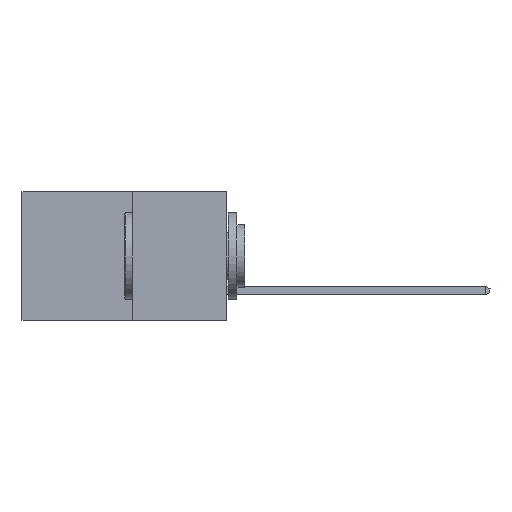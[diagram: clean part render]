
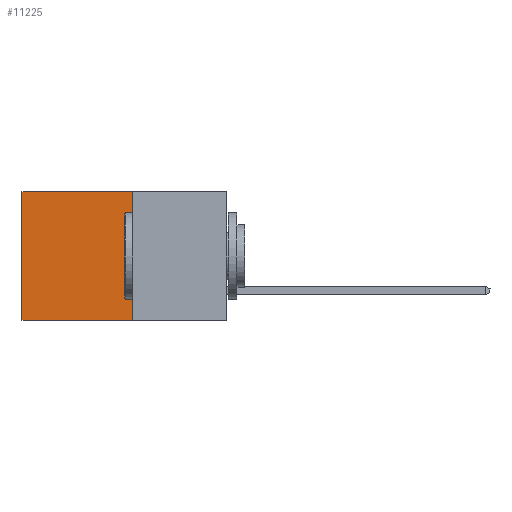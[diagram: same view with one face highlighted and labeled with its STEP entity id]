
A CAD part, left-side view. The second image highlights one B-rep face of the part: STEP entity #11225.
In plain terms, the highlighted planar face has unit normal (-1, 0, 0).
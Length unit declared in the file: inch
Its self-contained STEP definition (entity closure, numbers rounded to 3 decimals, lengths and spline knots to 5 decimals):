
#273 = EDGE_CURVE ( 'NONE', #6928, #7206, #2304, .T. ) ;
#679 = ORIENTED_EDGE ( 'NONE', *, *, #12634, .F. ) ;
#871 = EDGE_CURVE ( 'NONE', #11242, #6928, #12671, .T. ) ;
#1134 = AXIS2_PLACEMENT_3D ( 'NONE', #4849, #5871, #12575 ) ;
#1593 = LINE ( 'NONE', #10690, #6642 ) ;
#2304 = LINE ( 'NONE', #9283, #12414 ) ;
#3019 = LINE ( 'NONE', #3450, #8004 ) ;
#3258 = DIRECTION ( 'NONE',  ( 0., 0., -1. ) ) ;
#3450 = CARTESIAN_POINT ( 'NONE',  ( 0.277, 0.27, -0.37 ) ) ;
#3886 = CARTESIAN_POINT ( 'NONE',  ( 0.277, 0.27, 0. ) ) ;
#4463 = DIRECTION ( 'NONE',  ( 0., 1., 0. ) ) ;
#4674 = CARTESIAN_POINT ( 'NONE',  ( 0.277, 0.59, -0.37 ) ) ;
#4849 = CARTESIAN_POINT ( 'NONE',  ( 0.277, 0.27, -0.37 ) ) ;
#5871 = DIRECTION ( 'NONE',  ( 1., 0., 0. ) ) ;
#6015 = EDGE_LOOP ( 'NONE', ( #10899, #679, #6338, #11491 ) ) ;
#6338 = ORIENTED_EDGE ( 'NONE', *, *, #10645, .F. ) ;
#6536 = CARTESIAN_POINT ( 'NONE',  ( 0.277, 0.27, -0.37 ) ) ;
#6642 = VECTOR ( 'NONE', #12550, 39.37008 ) ;
#6742 = DIRECTION ( 'NONE',  ( 0., 1., 0. ) ) ;
#6928 = VERTEX_POINT ( 'NONE', #10574 ) ;
#7206 = VERTEX_POINT ( 'NONE', #4674 ) ;
#7909 = VECTOR ( 'NONE', #6742, 39.37008 ) ;
#8004 = VECTOR ( 'NONE', #4463, 39.37008 ) ;
#8428 = VERTEX_POINT ( 'NONE', #6536 ) ;
#8850 = CARTESIAN_POINT ( 'NONE',  ( 0.277, 0.27, 0. ) ) ;
#9283 = CARTESIAN_POINT ( 'NONE',  ( 0.277, 0.59, -0.37 ) ) ;
#9996 = FACE_OUTER_BOUND ( 'NONE', #6015, .T. ) ;
#10574 = CARTESIAN_POINT ( 'NONE',  ( 0.277, 0.59, 0. ) ) ;
#10645 = EDGE_CURVE ( 'NONE', #11242, #8428, #1593, .T. ) ;
#10690 = CARTESIAN_POINT ( 'NONE',  ( 0.277, 0.27, -0.37 ) ) ;
#10725 = PLANE ( 'NONE',  #1134 ) ;
#10899 = ORIENTED_EDGE ( 'NONE', *, *, #273, .T. ) ;
#11225 = ADVANCED_FACE ( 'NONE', ( #9996 ), #10725, .F. ) ;
#11242 = VERTEX_POINT ( 'NONE', #3886 ) ;
#11491 = ORIENTED_EDGE ( 'NONE', *, *, #871, .T. ) ;
#12414 = VECTOR ( 'NONE', #3258, 39.37008 ) ;
#12550 = DIRECTION ( 'NONE',  ( 0., 0., -1. ) ) ;
#12575 = DIRECTION ( 'NONE',  ( 0., 0., -1. ) ) ;
#12634 = EDGE_CURVE ( 'NONE', #8428, #7206, #3019, .T. ) ;
#12671 = LINE ( 'NONE', #8850, #7909 ) ;
